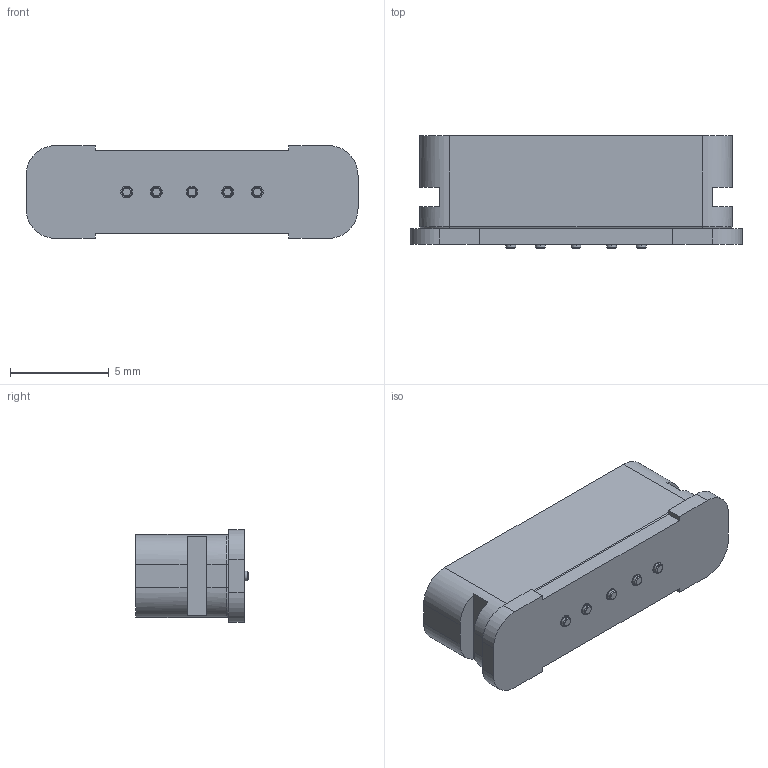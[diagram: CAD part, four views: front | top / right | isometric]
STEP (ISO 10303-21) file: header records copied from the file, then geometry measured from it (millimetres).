
FILE_DESCRIPTION (( 'STEP AP203' ), '1' );
FILE_NAME ('685-G0524P50110-NEW1.STEP', '2023-02-10T09:38:31', ( '' ), ( '' ), 'SwSTEP 2.0', 'SolidWorks 2020', '' );
FILE_SCHEMA (( 'CONFIG_CONTROL_DESIGN' ));
Length unit declared in the file: millimetre
Products named in the file (1): 685-G0524P50110-NEW1
Bounding box: 16.8 x 5.7 x 4.7 mm (x, y, z)
Volume: 336.4 mm3; surface area: 410.5 mm2
Topology: 11 solids, 11 shells, 137 faces, 302 edges, 189 vertices
Faces by surface type: plane 57, cylinder 54, cone 12, sphere 10, torus 4
Entity records: 3699 total; most frequent: DIRECTION 700, CARTESIAN_POINT 599, ORIENTED_EDGE 564, EDGE_CURVE 282, AXIS2_PLACEMENT_3D 280, VERTEX_POINT 179, EDGE_LOOP 149, CIRCLE 142
